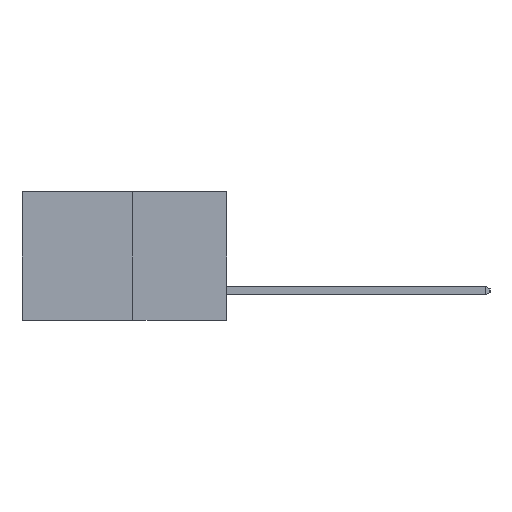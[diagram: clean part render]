
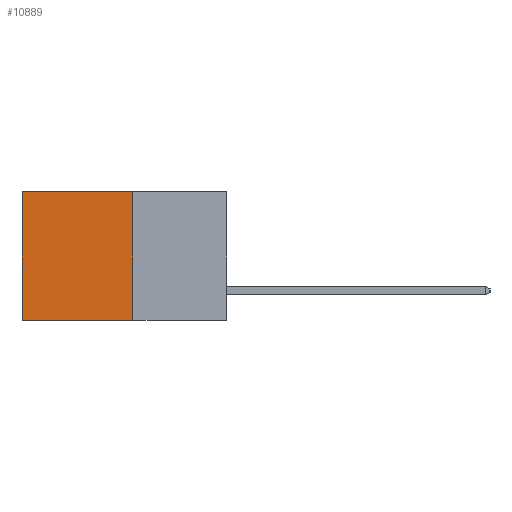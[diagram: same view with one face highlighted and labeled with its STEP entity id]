
A CAD part, left-side view. The second image highlights one B-rep face of the part: STEP entity #10889.
In plain terms, the highlighted planar face has unit normal (-1, 0, 0).
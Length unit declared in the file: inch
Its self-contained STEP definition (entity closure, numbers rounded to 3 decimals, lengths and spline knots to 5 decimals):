
#380 = VECTOR ( 'NONE', #21516, 39.37008 ) ;
#467 = AXIS2_PLACEMENT_3D ( 'NONE', #5583, #22493, #11262 ) ;
#1226 = CARTESIAN_POINT ( 'NONE',  ( 0.277, 0.27, 0. ) ) ;
#1321 = ORIENTED_EDGE ( 'NONE', *, *, #6243, .F. ) ;
#1666 = EDGE_LOOP ( 'NONE', ( #18403, #1321, #21119, #14900 ) ) ;
#2676 = VERTEX_POINT ( 'NONE', #11309 ) ;
#2691 = CARTESIAN_POINT ( 'NONE',  ( 0.277, 0.27, -0.37 ) ) ;
#3089 = EDGE_CURVE ( 'NONE', #10159, #24054, #7044, .T. ) ;
#3525 = DIRECTION ( 'NONE',  ( 0., 0., -1. ) ) ;
#4942 = CARTESIAN_POINT ( 'NONE',  ( 0.277, 0.27, -0.37 ) ) ;
#5583 = CARTESIAN_POINT ( 'NONE',  ( 0.277, 0.27, -0.37 ) ) ;
#6243 = EDGE_CURVE ( 'NONE', #24054, #2676, #20463, .T. ) ;
#6456 = VECTOR ( 'NONE', #22400, 39.37008 ) ;
#7044 = LINE ( 'NONE', #2691, #12612 ) ;
#7396 = CARTESIAN_POINT ( 'NONE',  ( 0.277, 0.27, 0. ) ) ;
#9408 = PLANE ( 'NONE',  #467 ) ;
#9936 = LINE ( 'NONE', #16682, #19947 ) ;
#10159 = VERTEX_POINT ( 'NONE', #1226 ) ;
#10291 = CARTESIAN_POINT ( 'NONE',  ( 0.277, 0.27, -0.37 ) ) ;
#10889 = ADVANCED_FACE ( 'NONE', ( #23237 ), #9408, .F. ) ;
#11262 = DIRECTION ( 'NONE',  ( 0., 0., -1. ) ) ;
#11309 = CARTESIAN_POINT ( 'NONE',  ( 0.277, 0.59, -0.37 ) ) ;
#12612 = VECTOR ( 'NONE', #19032, 39.37008 ) ;
#14900 = ORIENTED_EDGE ( 'NONE', *, *, #17539, .T. ) ;
#16427 = LINE ( 'NONE', #7396, #6456 ) ;
#16682 = CARTESIAN_POINT ( 'NONE',  ( 0.277, 0.59, -0.37 ) ) ;
#17539 = EDGE_CURVE ( 'NONE', #10159, #20909, #16427, .T. ) ;
#18403 = ORIENTED_EDGE ( 'NONE', *, *, #19794, .T. ) ;
#19032 = DIRECTION ( 'NONE',  ( 0., 0., -1. ) ) ;
#19794 = EDGE_CURVE ( 'NONE', #20909, #2676, #9936, .T. ) ;
#19947 = VECTOR ( 'NONE', #3525, 39.37008 ) ;
#20463 = LINE ( 'NONE', #10291, #380 ) ;
#20909 = VERTEX_POINT ( 'NONE', #20933 ) ;
#20933 = CARTESIAN_POINT ( 'NONE',  ( 0.277, 0.59, 0. ) ) ;
#21119 = ORIENTED_EDGE ( 'NONE', *, *, #3089, .F. ) ;
#21516 = DIRECTION ( 'NONE',  ( 0., 1., 0. ) ) ;
#22400 = DIRECTION ( 'NONE',  ( 0., 1., 0. ) ) ;
#22493 = DIRECTION ( 'NONE',  ( 1., 0., 0. ) ) ;
#23237 = FACE_OUTER_BOUND ( 'NONE', #1666, .T. ) ;
#24054 = VERTEX_POINT ( 'NONE', #4942 ) ;
